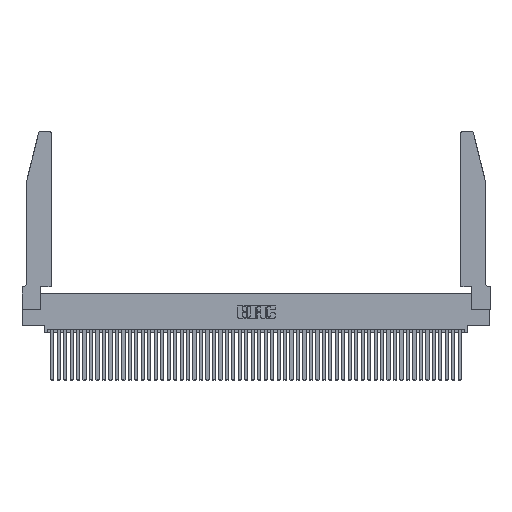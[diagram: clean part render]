
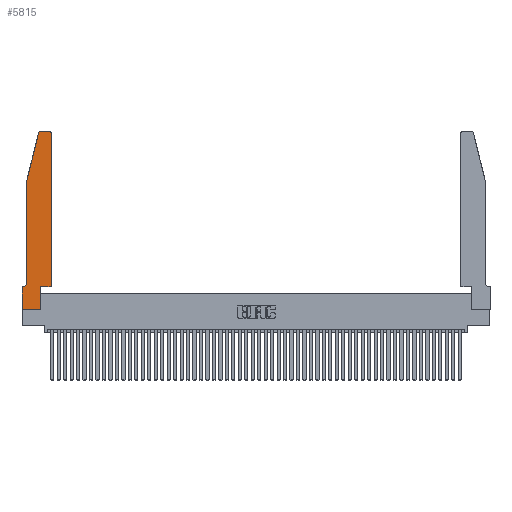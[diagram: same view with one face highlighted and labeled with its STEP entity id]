
A CAD part, top view. The second image highlights one B-rep face of the part: STEP entity #5815.
In plain terms, the highlighted planar face has unit normal (0, 0, 1).
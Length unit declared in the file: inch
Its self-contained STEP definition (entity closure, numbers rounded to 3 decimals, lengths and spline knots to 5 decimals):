
#245 = LINE ( 'NONE', #50777, #21953 ) ;
#2570 = EDGE_CURVE ( 'NONE', #30247, #6147, #27401, .T. ) ;
#2599 = DIRECTION ( 'NONE',  ( 0., 0., -1. ) ) ;
#2726 = VERTEX_POINT ( 'NONE', #10704 ) ;
#4027 = CARTESIAN_POINT ( 'NONE',  ( 0.25487, 2.72718, 0.37 ) ) ;
#4196 = CARTESIAN_POINT ( 'NONE',  ( 0.4505, 0.35, 0.37 ) ) ;
#4477 = LINE ( 'NONE', #48605, #24784 ) ;
#4897 = ORIENTED_EDGE ( 'NONE', *, *, #15295, .T. ) ;
#5457 = VERTEX_POINT ( 'NONE', #7312 ) ;
#5635 = EDGE_CURVE ( 'NONE', #2726, #18220, #47550, .T. ) ;
#5815 = ADVANCED_FACE ( 'NONE', ( #18971 ), #37397, .T. ) ;
#6147 = VERTEX_POINT ( 'NONE', #15846 ) ;
#7312 = CARTESIAN_POINT ( 'NONE',  ( 0.284, 2.75, 0.37 ) ) ;
#8313 = VECTOR ( 'NONE', #46455, 39.37008 ) ;
#8597 = ORIENTED_EDGE ( 'NONE', *, *, #16632, .T. ) ;
#9382 = VECTOR ( 'NONE', #36595, 39.37008 ) ;
#9604 = ORIENTED_EDGE ( 'NONE', *, *, #17905, .T. ) ;
#9803 = CARTESIAN_POINT ( 'NONE',  ( 0.4505, 0.35, 0.37 ) ) ;
#9943 = CARTESIAN_POINT ( 'NONE',  ( 0., 0.35, 0.37 ) ) ;
#10387 = VERTEX_POINT ( 'NONE', #29805 ) ;
#10704 = CARTESIAN_POINT ( 'NONE',  ( 0.0755, 2., 0.37 ) ) ;
#11115 = CARTESIAN_POINT ( 'NONE',  ( 0.4205, 2.72, 0.37 ) ) ;
#13657 = VECTOR ( 'NONE', #14123, 39.37008 ) ;
#13711 = ORIENTED_EDGE ( 'NONE', *, *, #14224, .T. ) ;
#13968 = AXIS2_PLACEMENT_3D ( 'NONE', #43985, #20245, #47972 ) ;
#14123 = DIRECTION ( 'NONE',  ( -1., 0., 0. ) ) ;
#14224 = EDGE_CURVE ( 'NONE', #21408, #5457, #23048, .T. ) ;
#15215 = DIRECTION ( 'NONE',  ( 1., 0., 0. ) ) ;
#15295 = EDGE_CURVE ( 'NONE', #41809, #10387, #4477, .T. ) ;
#15846 = CARTESIAN_POINT ( 'NONE',  ( 0.4505, 2.72, 0.37 ) ) ;
#16148 = VERTEX_POINT ( 'NONE', #32884 ) ;
#16597 = DIRECTION ( 'NONE',  ( 0., -1., 0. ) ) ;
#16632 = EDGE_CURVE ( 'NONE', #46261, #2726, #48920, .T. ) ;
#16793 = VECTOR ( 'NONE', #17955, 39.37008 ) ;
#16795 = CARTESIAN_POINT ( 'NONE',  ( 0.4505, 0.35, 0.37 ) ) ;
#17032 = EDGE_CURVE ( 'NONE', #18220, #31006, #38256, .T. ) ;
#17630 = AXIS2_PLACEMENT_3D ( 'NONE', #41392, #45378, #21675 ) ;
#17905 = EDGE_CURVE ( 'NONE', #31006, #41809, #19606, .T. ) ;
#17955 = DIRECTION ( 'NONE',  ( 0., 1., 0. ) ) ;
#18220 = VERTEX_POINT ( 'NONE', #34750 ) ;
#18570 = EDGE_CURVE ( 'NONE', #16148, #30247, #41226, .T. ) ;
#18694 = CARTESIAN_POINT ( 'NONE',  ( 0., 0., 0.37 ) ) ;
#18971 = FACE_OUTER_BOUND ( 'NONE', #30480, .T. ) ;
#19606 = LINE ( 'NONE', #21083, #50011 ) ;
#19794 = ORIENTED_EDGE ( 'NONE', *, *, #2570, .T. ) ;
#20245 = DIRECTION ( 'NONE',  ( 0., 0., 1. ) ) ;
#20647 = AXIS2_PLACEMENT_3D ( 'NONE', #26859, #2599, #30872 ) ;
#21083 = CARTESIAN_POINT ( 'NONE',  ( 0.0755, 0.35, 0.37 ) ) ;
#21408 = VERTEX_POINT ( 'NONE', #24895 ) ;
#21675 = DIRECTION ( 'NONE',  ( 1., 0., 0. ) ) ;
#21953 = VECTOR ( 'NONE', #27027, 39.37008 ) ;
#22584 = ORIENTED_EDGE ( 'NONE', *, *, #41494, .T. ) ;
#23048 = LINE ( 'NONE', #26147, #13657 ) ;
#24784 = VECTOR ( 'NONE', #44608, 39.37008 ) ;
#24895 = CARTESIAN_POINT ( 'NONE',  ( 0.4205, 2.75, 0.37 ) ) ;
#25068 = DIRECTION ( 'NONE',  ( -1., 0., 0. ) ) ;
#25307 = CIRCLE ( 'NONE', #13968, 0.03 ) ;
#26147 = CARTESIAN_POINT ( 'NONE',  ( 0.2605, 2.75, 0.37 ) ) ;
#26859 = CARTESIAN_POINT ( 'NONE',  ( 0.0055, 0.42, 0.37 ) ) ;
#27027 = DIRECTION ( 'NONE',  ( 0., 1., 0. ) ) ;
#27128 = ORIENTED_EDGE ( 'NONE', *, *, #17032, .T. ) ;
#27401 = LINE ( 'NONE', #9803, #16793 ) ;
#28322 = ORIENTED_EDGE ( 'NONE', *, *, #46070, .T. ) ;
#29805 = CARTESIAN_POINT ( 'NONE',  ( 0., 0., 0.37 ) ) ;
#30247 = VERTEX_POINT ( 'NONE', #4196 ) ;
#30437 = CARTESIAN_POINT ( 'NONE',  ( 0.0055, 0.35, 0.37 ) ) ;
#30480 = EDGE_LOOP ( 'NONE', ( #13711, #22584, #8597, #38220, #27128, #9604, #4897, #49765, #50617, #40154, #19794, #28322 ) ) ;
#30872 = DIRECTION ( 'NONE',  ( -1., 0., 0. ) ) ;
#31006 = VERTEX_POINT ( 'NONE', #30437 ) ;
#32884 = CARTESIAN_POINT ( 'NONE',  ( 0.2865, 0.35, 0.37 ) ) ;
#34715 = EDGE_CURVE ( 'NONE', #10387, #47057, #49547, .T. ) ;
#34750 = CARTESIAN_POINT ( 'NONE',  ( 0.0755, 0.42, 0.37 ) ) ;
#36595 = DIRECTION ( 'NONE',  ( 1., 0., 0. ) ) ;
#37093 = VECTOR ( 'NONE', #43707, 39.37008 ) ;
#37397 = PLANE ( 'NONE',  #17630 ) ;
#37521 = EDGE_CURVE ( 'NONE', #47057, #16148, #245, .T. ) ;
#38220 = ORIENTED_EDGE ( 'NONE', *, *, #5635, .T. ) ;
#38256 = CIRCLE ( 'NONE', #20647, 0.07 ) ;
#38362 = AXIS2_PLACEMENT_3D ( 'NONE', #11115, #38984, #15215 ) ;
#38984 = DIRECTION ( 'NONE',  ( 0., 0., 1. ) ) ;
#39115 = CIRCLE ( 'NONE', #38362, 0.03 ) ;
#39517 = CARTESIAN_POINT ( 'NONE',  ( 0.0755, 2., 0.37 ) ) ;
#40154 = ORIENTED_EDGE ( 'NONE', *, *, #18570, .T. ) ;
#41226 = LINE ( 'NONE', #16795, #9382 ) ;
#41392 = CARTESIAN_POINT ( 'NONE',  ( 0., 0.35, 0.37 ) ) ;
#41494 = EDGE_CURVE ( 'NONE', #5457, #46261, #25307, .T. ) ;
#41809 = VERTEX_POINT ( 'NONE', #9943 ) ;
#43707 = DIRECTION ( 'NONE',  ( -0.239, -0.971, 0. ) ) ;
#43985 = CARTESIAN_POINT ( 'NONE',  ( 0.284, 2.72, 0.37 ) ) ;
#44206 = CARTESIAN_POINT ( 'NONE',  ( 0.0755, 2., 0.37 ) ) ;
#44608 = DIRECTION ( 'NONE',  ( 0., -1., 0. ) ) ;
#45378 = DIRECTION ( 'NONE',  ( 0., 0., 1. ) ) ;
#46070 = EDGE_CURVE ( 'NONE', #6147, #21408, #39115, .T. ) ;
#46261 = VERTEX_POINT ( 'NONE', #4027 ) ;
#46300 = VECTOR ( 'NONE', #16597, 39.37008 ) ;
#46455 = DIRECTION ( 'NONE',  ( 1., 0., 0. ) ) ;
#47057 = VERTEX_POINT ( 'NONE', #48122 ) ;
#47550 = LINE ( 'NONE', #44206, #46300 ) ;
#47972 = DIRECTION ( 'NONE',  ( 1., 0., 0. ) ) ;
#48122 = CARTESIAN_POINT ( 'NONE',  ( 0.2865, 0., 0.37 ) ) ;
#48605 = CARTESIAN_POINT ( 'NONE',  ( 0., 0., 0.37 ) ) ;
#48920 = LINE ( 'NONE', #39517, #37093 ) ;
#49547 = LINE ( 'NONE', #18694, #8313 ) ;
#49765 = ORIENTED_EDGE ( 'NONE', *, *, #34715, .T. ) ;
#50011 = VECTOR ( 'NONE', #25068, 39.37008 ) ;
#50617 = ORIENTED_EDGE ( 'NONE', *, *, #37521, .T. ) ;
#50777 = CARTESIAN_POINT ( 'NONE',  ( 0.2865, 0.35, 0.37 ) ) ;
